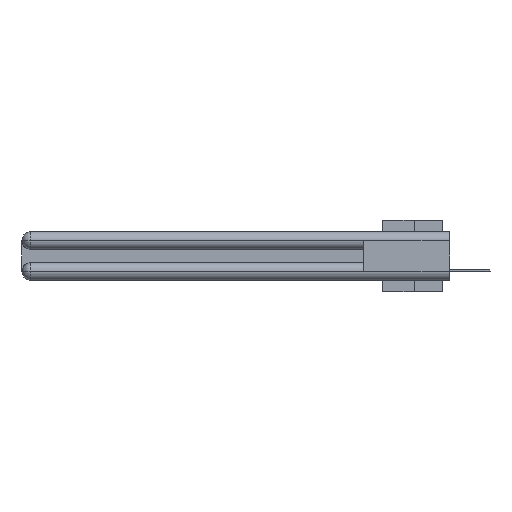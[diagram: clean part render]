
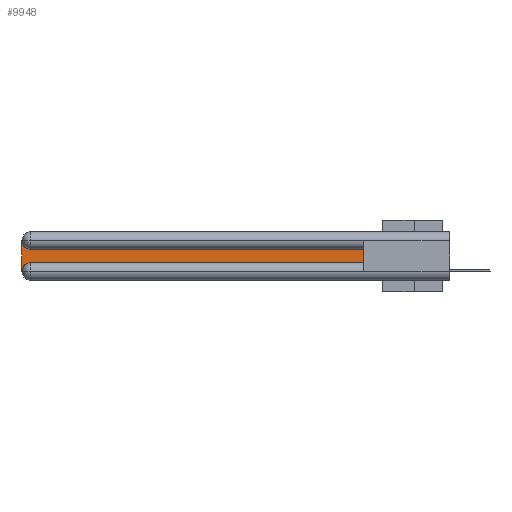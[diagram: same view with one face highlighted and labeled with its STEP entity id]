
A CAD part, left-side view. The second image highlights one B-rep face of the part: STEP entity #9948.
In plain terms, the highlighted planar face has unit normal (-1, 0, 0).
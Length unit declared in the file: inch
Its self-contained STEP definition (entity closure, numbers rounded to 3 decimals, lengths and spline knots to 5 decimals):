
#144 = CARTESIAN_POINT ( 'NONE',  ( 0.075, 0.6, -0.2175 ) ) ;
#214 = EDGE_CURVE ( 'NONE', #21471, #28717, #4158, .T. ) ;
#1411 = CARTESIAN_POINT ( 'NONE',  ( 0.075, 0.6, -0.2175 ) ) ;
#2122 = ORIENTED_EDGE ( 'NONE', *, *, #21622, .T. ) ;
#2774 = ORIENTED_EDGE ( 'NONE', *, *, #214, .T. ) ;
#3450 = ORIENTED_EDGE ( 'NONE', *, *, #20151, .T. ) ;
#3633 = DIRECTION ( 'NONE',  ( 0., 0., 1. ) ) ;
#4158 = CIRCLE ( 'NONE', #25648, 0.06 ) ;
#4307 = EDGE_CURVE ( 'NONE', #27420, #22650, #11822, .T. ) ;
#4483 = DIRECTION ( 'NONE',  ( 0., 0., -1. ) ) ;
#8175 = EDGE_CURVE ( 'NONE', #28717, #27420, #30379, .T. ) ;
#9066 = AXIS2_PLACEMENT_3D ( 'NONE', #10912, #13466, #4483 ) ;
#9845 = DIRECTION ( 'NONE',  ( 0., 0., -1. ) ) ;
#9948 = ADVANCED_FACE ( 'NONE', ( #33426 ), #19093, .F. ) ;
#10861 = DIRECTION ( 'NONE',  ( 0., 0., -1. ) ) ;
#10912 = CARTESIAN_POINT ( 'NONE',  ( 0.075, 3., -0.1225 ) ) ;
#11822 = CIRCLE ( 'NONE', #28855, 0.06 ) ;
#12346 = VECTOR ( 'NONE', #26761, 39.37008 ) ;
#13261 = DIRECTION ( 'NONE',  ( 0., 1., 0. ) ) ;
#13466 = DIRECTION ( 'NONE',  ( 1., 0., 0. ) ) ;
#14232 = ORIENTED_EDGE ( 'NONE', *, *, #8175, .T. ) ;
#14327 = CARTESIAN_POINT ( 'NONE',  ( 0.075, 0.6, -0.1225 ) ) ;
#14668 = DIRECTION ( 'NONE',  ( 0., 0., -1. ) ) ;
#15438 = VECTOR ( 'NONE', #13261, 39.37008 ) ;
#15847 = VERTEX_POINT ( 'NONE', #1411 ) ;
#17455 = LINE ( 'NONE', #36134, #28164 ) ;
#18042 = CARTESIAN_POINT ( 'NONE',  ( 0.075, 3., -0.2175 ) ) ;
#19093 = PLANE ( 'NONE',  #9066 ) ;
#19718 = EDGE_LOOP ( 'NONE', ( #2122, #2774, #14232, #21114, #28116, #3450 ) ) ;
#19758 = VECTOR ( 'NONE', #14668, 39.37008 ) ;
#20151 = EDGE_CURVE ( 'NONE', #15847, #26385, #17455, .T. ) ;
#21114 = ORIENTED_EDGE ( 'NONE', *, *, #4307, .T. ) ;
#21471 = VERTEX_POINT ( 'NONE', #24076 ) ;
#21622 = EDGE_CURVE ( 'NONE', #26385, #21471, #35552, .T. ) ;
#21924 = CARTESIAN_POINT ( 'NONE',  ( 0.075, 3., -0.2775 ) ) ;
#22020 = CARTESIAN_POINT ( 'NONE',  ( 0.075, 0.6, -0.1225 ) ) ;
#22650 = VERTEX_POINT ( 'NONE', #36040 ) ;
#23493 = CARTESIAN_POINT ( 'NONE',  ( 0.075, 3., -0.0625 ) ) ;
#24076 = CARTESIAN_POINT ( 'NONE',  ( 0.075, 2.94, -0.1225 ) ) ;
#25648 = AXIS2_PLACEMENT_3D ( 'NONE', #27216, #27464, #9845 ) ;
#25976 = LINE ( 'NONE', #144, #12346 ) ;
#26385 = VERTEX_POINT ( 'NONE', #14327 ) ;
#26761 = DIRECTION ( 'NONE',  ( 0., -1., 0. ) ) ;
#27216 = CARTESIAN_POINT ( 'NONE',  ( 0.075, 2.94, -0.0625 ) ) ;
#27420 = VERTEX_POINT ( 'NONE', #21924 ) ;
#27464 = DIRECTION ( 'NONE',  ( 1., 0., 0. ) ) ;
#28116 = ORIENTED_EDGE ( 'NONE', *, *, #30636, .T. ) ;
#28164 = VECTOR ( 'NONE', #3633, 39.37008 ) ;
#28717 = VERTEX_POINT ( 'NONE', #23493 ) ;
#28855 = AXIS2_PLACEMENT_3D ( 'NONE', #32192, #31820, #10861 ) ;
#30379 = LINE ( 'NONE', #18042, #19758 ) ;
#30636 = EDGE_CURVE ( 'NONE', #22650, #15847, #25976, .T. ) ;
#31820 = DIRECTION ( 'NONE',  ( 1., 0., 0. ) ) ;
#32192 = CARTESIAN_POINT ( 'NONE',  ( 0.075, 2.94, -0.2775 ) ) ;
#33426 = FACE_OUTER_BOUND ( 'NONE', #19718, .T. ) ;
#35552 = LINE ( 'NONE', #22020, #15438 ) ;
#36040 = CARTESIAN_POINT ( 'NONE',  ( 0.075, 2.94, -0.2175 ) ) ;
#36134 = CARTESIAN_POINT ( 'NONE',  ( 0.075, 0.6, -0.2175 ) ) ;
